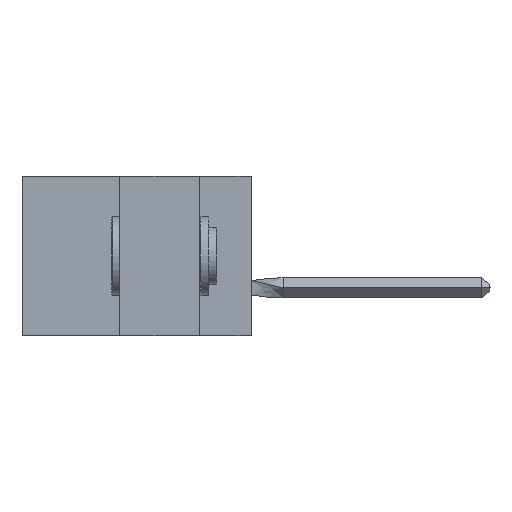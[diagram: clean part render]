
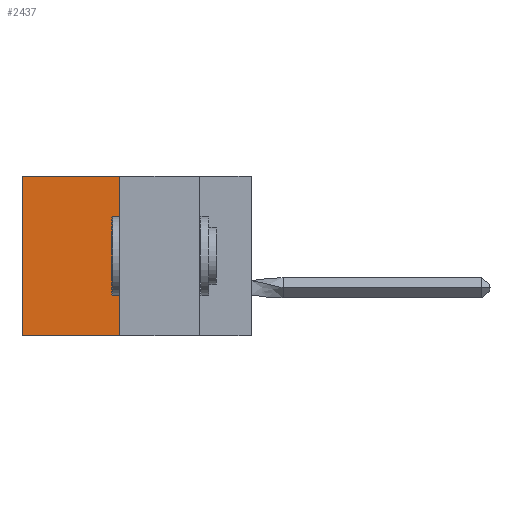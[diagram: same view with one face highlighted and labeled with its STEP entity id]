
A CAD part, left-side view. The second image highlights one B-rep face of the part: STEP entity #2437.
In plain terms, the highlighted planar face has unit normal (-1, 0, 0).
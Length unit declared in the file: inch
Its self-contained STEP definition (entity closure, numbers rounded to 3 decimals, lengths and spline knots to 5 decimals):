
#663 = DIRECTION ( 'NONE',  ( 0., 1., 0. ) ) ;
#693 = VERTEX_POINT ( 'NONE', #6098 ) ;
#2317 = LINE ( 'NONE', #5063, #3195 ) ;
#2437 = ADVANCED_FACE ( 'NONE', ( #12862 ), #19929, .F. ) ;
#2602 = EDGE_CURVE ( 'NONE', #2972, #14789, #4601, .T. ) ;
#2822 = VECTOR ( 'NONE', #19312, 39.37008 ) ;
#2929 = DIRECTION ( 'NONE',  ( 1., 0., 0. ) ) ;
#2943 = ORIENTED_EDGE ( 'NONE', *, *, #6886, .F. ) ;
#2972 = VERTEX_POINT ( 'NONE', #14722 ) ;
#3195 = VECTOR ( 'NONE', #14261, 39.37008 ) ;
#4601 = LINE ( 'NONE', #11165, #18825 ) ;
#4844 = CARTESIAN_POINT ( 'NONE',  ( 0.305, 0.413, -0.5 ) ) ;
#4953 = VECTOR ( 'NONE', #663, 39.37008 ) ;
#5063 = CARTESIAN_POINT ( 'NONE',  ( 0.305, 0.413, -0.5 ) ) ;
#5825 = LINE ( 'NONE', #6183, #4953 ) ;
#6033 = ORIENTED_EDGE ( 'NONE', *, *, #19955, .T. ) ;
#6098 = CARTESIAN_POINT ( 'NONE',  ( 0.305, 0.72, 0. ) ) ;
#6183 = CARTESIAN_POINT ( 'NONE',  ( 0.305, 0.413, 0. ) ) ;
#6816 = EDGE_LOOP ( 'NONE', ( #7203, #2943, #14149, #6033 ) ) ;
#6886 = EDGE_CURVE ( 'NONE', #14789, #7951, #2317, .T. ) ;
#7203 = ORIENTED_EDGE ( 'NONE', *, *, #8885, .T. ) ;
#7951 = VERTEX_POINT ( 'NONE', #18107 ) ;
#8656 = CARTESIAN_POINT ( 'NONE',  ( 0.305, 0.413, -0.5 ) ) ;
#8885 = EDGE_CURVE ( 'NONE', #693, #7951, #19740, .T. ) ;
#11165 = CARTESIAN_POINT ( 'NONE',  ( 0.305, 0.413, -0.5 ) ) ;
#12862 = FACE_OUTER_BOUND ( 'NONE', #6816, .T. ) ;
#14149 = ORIENTED_EDGE ( 'NONE', *, *, #2602, .F. ) ;
#14261 = DIRECTION ( 'NONE',  ( 0., 1., 0. ) ) ;
#14517 = DIRECTION ( 'NONE',  ( 0., 0., -1. ) ) ;
#14722 = CARTESIAN_POINT ( 'NONE',  ( 0.305, 0.413, 0. ) ) ;
#14789 = VERTEX_POINT ( 'NONE', #8656 ) ;
#17399 = CARTESIAN_POINT ( 'NONE',  ( 0.305, 0.72, -0.5 ) ) ;
#18107 = CARTESIAN_POINT ( 'NONE',  ( 0.305, 0.72, -0.5 ) ) ;
#18597 = DIRECTION ( 'NONE',  ( 0., 0., -1. ) ) ;
#18825 = VECTOR ( 'NONE', #18597, 39.37008 ) ;
#19312 = DIRECTION ( 'NONE',  ( 0., 0., -1. ) ) ;
#19471 = AXIS2_PLACEMENT_3D ( 'NONE', #4844, #2929, #14517 ) ;
#19740 = LINE ( 'NONE', #17399, #2822 ) ;
#19929 = PLANE ( 'NONE',  #19471 ) ;
#19955 = EDGE_CURVE ( 'NONE', #2972, #693, #5825, .T. ) ;
